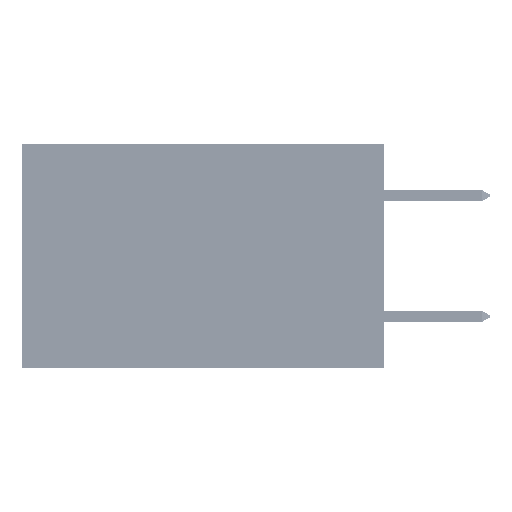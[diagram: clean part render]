
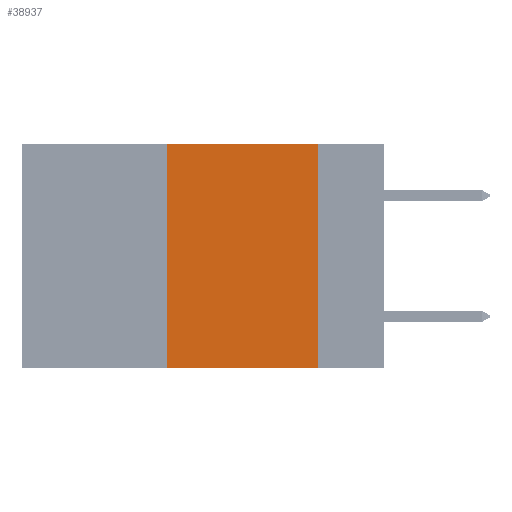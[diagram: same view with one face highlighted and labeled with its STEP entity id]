
A CAD part, left-side view. The second image highlights one B-rep face of the part: STEP entity #38937.
In plain terms, the highlighted planar face has unit normal (-1, 0, 0).
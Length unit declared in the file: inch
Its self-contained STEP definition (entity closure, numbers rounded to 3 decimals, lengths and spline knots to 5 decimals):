
#1766 = VECTOR ( 'NONE', #35159, 39.37008 ) ;
#2095 = CARTESIAN_POINT ( 'NONE',  ( 0., 0.36, 0. ) ) ;
#2958 = VECTOR ( 'NONE', #43991, 39.37008 ) ;
#5659 = EDGE_CURVE ( 'NONE', #27143, #18716, #23093, .T. ) ;
#5937 = CARTESIAN_POINT ( 'NONE',  ( 0., 0.6, 0. ) ) ;
#6306 = ORIENTED_EDGE ( 'NONE', *, *, #13161, .F. ) ;
#10115 = LINE ( 'NONE', #27684, #1766 ) ;
#10411 = CARTESIAN_POINT ( 'NONE',  ( 0., 0.11, 0. ) ) ;
#10546 = ORIENTED_EDGE ( 'NONE', *, *, #5659, .T. ) ;
#10662 = VERTEX_POINT ( 'NONE', #2095 ) ;
#13161 = EDGE_CURVE ( 'NONE', #27143, #10662, #10115, .T. ) ;
#13555 = VECTOR ( 'NONE', #47889, 39.37008 ) ;
#14808 = EDGE_CURVE ( 'NONE', #10662, #15462, #30823, .T. ) ;
#15462 = VERTEX_POINT ( 'NONE', #10411 ) ;
#16326 = ORIENTED_EDGE ( 'NONE', *, *, #41463, .F. ) ;
#18130 = CARTESIAN_POINT ( 'NONE',  ( 0., 0.6, 0. ) ) ;
#18497 = AXIS2_PLACEMENT_3D ( 'NONE', #5937, #40243, #39765 ) ;
#18716 = VERTEX_POINT ( 'NONE', #36924 ) ;
#20927 = PLANE ( 'NONE',  #18497 ) ;
#23093 = LINE ( 'NONE', #28760, #13555 ) ;
#25058 = EDGE_LOOP ( 'NONE', ( #16326, #26686, #6306, #10546 ) ) ;
#26686 = ORIENTED_EDGE ( 'NONE', *, *, #14808, .F. ) ;
#27143 = VERTEX_POINT ( 'NONE', #43867 ) ;
#27684 = CARTESIAN_POINT ( 'NONE',  ( 0., 0.36, 0. ) ) ;
#28760 = CARTESIAN_POINT ( 'NONE',  ( 0., 0.6, -0.37 ) ) ;
#30823 = LINE ( 'NONE', #18130, #33778 ) ;
#33778 = VECTOR ( 'NONE', #48271, 39.37008 ) ;
#35159 = DIRECTION ( 'NONE',  ( 0., 0., 1. ) ) ;
#36924 = CARTESIAN_POINT ( 'NONE',  ( 0., 0.11, -0.37 ) ) ;
#38937 = ADVANCED_FACE ( 'NONE', ( #48879 ), #20927, .F. ) ;
#39664 = CARTESIAN_POINT ( 'NONE',  ( 0., 0.11, 0. ) ) ;
#39765 = DIRECTION ( 'NONE',  ( 0., 0., -1. ) ) ;
#40243 = DIRECTION ( 'NONE',  ( 1., 0., 0. ) ) ;
#41463 = EDGE_CURVE ( 'NONE', #15462, #18716, #44704, .T. ) ;
#43867 = CARTESIAN_POINT ( 'NONE',  ( 0., 0.36, -0.37 ) ) ;
#43991 = DIRECTION ( 'NONE',  ( 0., 0., -1. ) ) ;
#44704 = LINE ( 'NONE', #39664, #2958 ) ;
#47889 = DIRECTION ( 'NONE',  ( 0., -1., 0. ) ) ;
#48271 = DIRECTION ( 'NONE',  ( 0., -1., 0. ) ) ;
#48879 = FACE_OUTER_BOUND ( 'NONE', #25058, .T. ) ;
